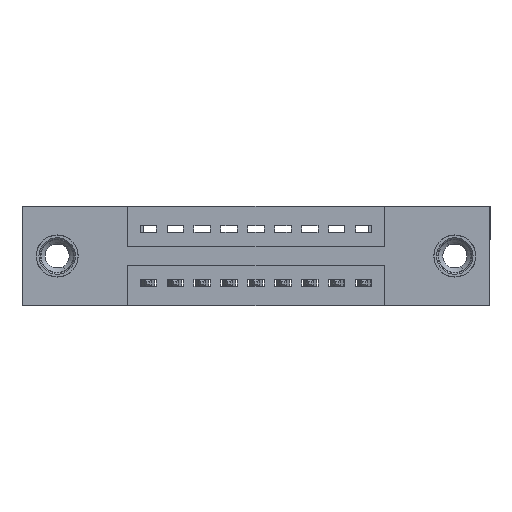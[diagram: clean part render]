
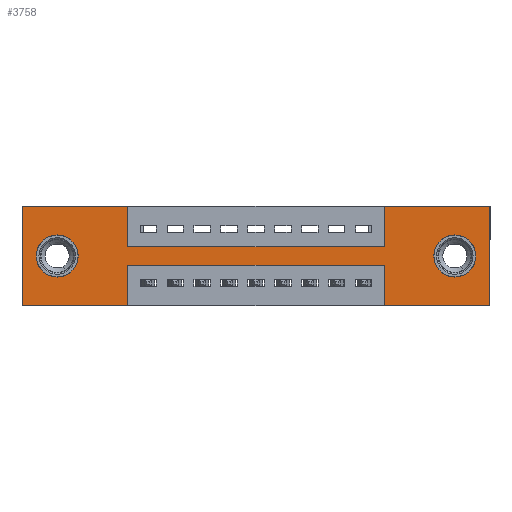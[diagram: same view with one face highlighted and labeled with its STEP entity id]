
A CAD part, front view. The second image highlights one B-rep face of the part: STEP entity #3758.
In plain terms, the highlighted planar face has unit normal (0, -1, 0).
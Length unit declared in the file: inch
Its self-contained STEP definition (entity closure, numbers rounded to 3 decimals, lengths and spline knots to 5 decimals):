
#44 = VECTOR ( 'NONE', #261, 39.37008 ) ;
#188 = VERTEX_POINT ( 'NONE', #5067 ) ;
#201 = EDGE_CURVE ( 'NONE', #7228, #4524, #6579, .T. ) ;
#225 = EDGE_CURVE ( 'NONE', #1121, #188, #7376, .T. ) ;
#253 = ORIENTED_EDGE ( 'NONE', *, *, #12209, .F. ) ;
#261 = DIRECTION ( 'NONE',  ( 0., 0., -1. ) ) ;
#304 = VERTEX_POINT ( 'NONE', #8446 ) ;
#416 = EDGE_CURVE ( 'NONE', #8986, #6465, #934, .T. ) ;
#478 = CARTESIAN_POINT ( 'NONE',  ( 0., 0., 0. ) ) ;
#480 = DIRECTION ( 'NONE',  ( 1., 0., 0. ) ) ;
#505 = LINE ( 'NONE', #9647, #12288 ) ;
#551 = ORIENTED_EDGE ( 'NONE', *, *, #8954, .F. ) ;
#598 = ORIENTED_EDGE ( 'NONE', *, *, #416, .T. ) ;
#721 = CARTESIAN_POINT ( 'NONE',  ( 0.3925, 0., -0.15 ) ) ;
#870 = ORIENTED_EDGE ( 'NONE', *, *, #201, .F. ) ;
#888 = EDGE_CURVE ( 'NONE', #2505, #5016, #10098, .T. ) ;
#934 = CIRCLE ( 'NONE', #12298, 0.078 ) ;
#1121 = VERTEX_POINT ( 'NONE', #9405 ) ;
#1177 = LINE ( 'NONE', #2884, #6327 ) ;
#1178 = EDGE_CURVE ( 'NONE', #2474, #5513, #10087, .T. ) ;
#1232 = CARTESIAN_POINT ( 'NONE',  ( 1.3425, 0., -0.15 ) ) ;
#1363 = LINE ( 'NONE', #12987, #12840 ) ;
#1561 = DIRECTION ( 'NONE',  ( 0., 0., 1. ) ) ;
#1634 = ORIENTED_EDGE ( 'NONE', *, *, #2794, .F. ) ;
#1692 = DIRECTION ( 'NONE',  ( 0., 0., -1. ) ) ;
#1800 = LINE ( 'NONE', #11561, #6954 ) ;
#2004 = DIRECTION ( 'NONE',  ( 0., 0., -1. ) ) ;
#2189 = DIRECTION ( 'NONE',  ( 0., 1., 0. ) ) ;
#2382 = AXIS2_PLACEMENT_3D ( 'NONE', #7420, #2189, #8302 ) ;
#2464 = EDGE_CURVE ( 'NONE', #6863, #6391, #1363, .T. ) ;
#2474 = VERTEX_POINT ( 'NONE', #10670 ) ;
#2505 = VERTEX_POINT ( 'NONE', #6942 ) ;
#2624 = LINE ( 'NONE', #8159, #13284 ) ;
#2680 = ORIENTED_EDGE ( 'NONE', *, *, #2464, .F. ) ;
#2794 = EDGE_CURVE ( 'NONE', #12512, #304, #3774, .T. ) ;
#2876 = CARTESIAN_POINT ( 'NONE',  ( 0.3925, 0., -0.37 ) ) ;
#2884 = CARTESIAN_POINT ( 'NONE',  ( 0., 0., 0. ) ) ;
#2957 = CARTESIAN_POINT ( 'NONE',  ( 0., 0., -0.37 ) ) ;
#3030 = DIRECTION ( 'NONE',  ( 0., 0., -1. ) ) ;
#3136 = VECTOR ( 'NONE', #8350, 39.37008 ) ;
#3281 = ORIENTED_EDGE ( 'NONE', *, *, #9114, .F. ) ;
#3407 = CIRCLE ( 'NONE', #9245, 0.078 ) ;
#3470 = CARTESIAN_POINT ( 'NONE',  ( 0., 0., -0.37 ) ) ;
#3683 = CARTESIAN_POINT ( 'NONE',  ( 1.605, 0., -0.185 ) ) ;
#3758 = ADVANCED_FACE ( 'NONE', ( #7115, #6798, #6649 ), #9208, .T. ) ;
#3774 = LINE ( 'NONE', #12649, #44 ) ;
#3925 = EDGE_CURVE ( 'NONE', #6465, #8986, #5951, .T. ) ;
#3928 = CARTESIAN_POINT ( 'NONE',  ( 1.605, 0., -0.107 ) ) ;
#3933 = ORIENTED_EDGE ( 'NONE', *, *, #9561, .F. ) ;
#4000 = VECTOR ( 'NONE', #10602, 39.37008 ) ;
#4123 = CARTESIAN_POINT ( 'NONE',  ( 0., 0., 0. ) ) ;
#4333 = VECTOR ( 'NONE', #9748, 39.37008 ) ;
#4355 = CARTESIAN_POINT ( 'NONE',  ( 0.3925, 0., 0. ) ) ;
#4524 = VERTEX_POINT ( 'NONE', #8348 ) ;
#4601 = CARTESIAN_POINT ( 'NONE',  ( 0.3925, 0., -0.22 ) ) ;
#4746 = CARTESIAN_POINT ( 'NONE',  ( 1.605, 0., -0.185 ) ) ;
#4803 = CARTESIAN_POINT ( 'NONE',  ( 0.13, 0., -0.185 ) ) ;
#4820 = LINE ( 'NONE', #2876, #8346 ) ;
#5016 = VERTEX_POINT ( 'NONE', #3928 ) ;
#5031 = LINE ( 'NONE', #721, #9381 ) ;
#5067 = CARTESIAN_POINT ( 'NONE',  ( 0., 0., -0.37 ) ) ;
#5081 = DIRECTION ( 'NONE',  ( 0., 0., -1. ) ) ;
#5088 = DIRECTION ( 'NONE',  ( 1., 0., 0. ) ) ;
#5110 = VECTOR ( 'NONE', #1561, 39.37008 ) ;
#5188 = EDGE_LOOP ( 'NONE', ( #9864, #8429 ) ) ;
#5513 = VERTEX_POINT ( 'NONE', #7099 ) ;
#5770 = DIRECTION ( 'NONE',  ( 0., 1., 0. ) ) ;
#5865 = AXIS2_PLACEMENT_3D ( 'NONE', #4746, #6835, #1692 ) ;
#5914 = DIRECTION ( 'NONE',  ( 1., 0., 0. ) ) ;
#5951 = CIRCLE ( 'NONE', #2382, 0.078 ) ;
#6327 = VECTOR ( 'NONE', #5088, 39.37008 ) ;
#6391 = VERTEX_POINT ( 'NONE', #9719 ) ;
#6465 = VERTEX_POINT ( 'NONE', #10808 ) ;
#6498 = EDGE_LOOP ( 'NONE', ( #598, #12131 ) ) ;
#6579 = LINE ( 'NONE', #4601, #4000 ) ;
#6613 = EDGE_CURVE ( 'NONE', #188, #6941, #13375, .T. ) ;
#6649 = FACE_OUTER_BOUND ( 'NONE', #7672, .T. ) ;
#6798 = FACE_BOUND ( 'NONE', #6498, .T. ) ;
#6835 = DIRECTION ( 'NONE',  ( 0., 1., 0. ) ) ;
#6863 = VERTEX_POINT ( 'NONE', #11289 ) ;
#6941 = VERTEX_POINT ( 'NONE', #4123 ) ;
#6942 = CARTESIAN_POINT ( 'NONE',  ( 1.605, 0., -0.263 ) ) ;
#6954 = VECTOR ( 'NONE', #12658, 39.37008 ) ;
#7099 = CARTESIAN_POINT ( 'NONE',  ( 1.3425, 0., -0.37 ) ) ;
#7115 = FACE_BOUND ( 'NONE', #5188, .T. ) ;
#7228 = VERTEX_POINT ( 'NONE', #7607 ) ;
#7376 = LINE ( 'NONE', #3470, #4333 ) ;
#7420 = CARTESIAN_POINT ( 'NONE',  ( 0.13, 0., -0.185 ) ) ;
#7607 = CARTESIAN_POINT ( 'NONE',  ( 1.3425, 0., -0.22 ) ) ;
#7672 = EDGE_LOOP ( 'NONE', ( #253, #870, #7832, #12107, #3933, #2680, #3281, #8566, #1634, #551, #10518, #7903 ) ) ;
#7832 = ORIENTED_EDGE ( 'NONE', *, *, #11456, .F. ) ;
#7903 = ORIENTED_EDGE ( 'NONE', *, *, #225, .F. ) ;
#8159 = CARTESIAN_POINT ( 'NONE',  ( 1.735, 0., 0. ) ) ;
#8302 = DIRECTION ( 'NONE',  ( 0., 0., 1. ) ) ;
#8346 = VECTOR ( 'NONE', #5081, 39.37008 ) ;
#8348 = CARTESIAN_POINT ( 'NONE',  ( 0.3925, 0., -0.22 ) ) ;
#8350 = DIRECTION ( 'NONE',  ( -1., 0., 0. ) ) ;
#8429 = ORIENTED_EDGE ( 'NONE', *, *, #888, .T. ) ;
#8446 = CARTESIAN_POINT ( 'NONE',  ( 0.3925, 0., -0.15 ) ) ;
#8566 = ORIENTED_EDGE ( 'NONE', *, *, #9412, .F. ) ;
#8755 = VERTEX_POINT ( 'NONE', #1232 ) ;
#8786 = DIRECTION ( 'NONE',  ( 0., 0., 1. ) ) ;
#8954 = EDGE_CURVE ( 'NONE', #6941, #12512, #1177, .T. ) ;
#8986 = VERTEX_POINT ( 'NONE', #11293 ) ;
#9114 = EDGE_CURVE ( 'NONE', #8755, #6863, #1800, .T. ) ;
#9208 = PLANE ( 'NONE',  #10697 ) ;
#9245 = AXIS2_PLACEMENT_3D ( 'NONE', #3683, #11915, #9806 ) ;
#9250 = DIRECTION ( 'NONE',  ( 0., -1., 0. ) ) ;
#9381 = VECTOR ( 'NONE', #5914, 39.37008 ) ;
#9405 = CARTESIAN_POINT ( 'NONE',  ( 0.3925, 0., -0.37 ) ) ;
#9412 = EDGE_CURVE ( 'NONE', #304, #8755, #5031, .T. ) ;
#9451 = CARTESIAN_POINT ( 'NONE',  ( 0., 0., -0.37 ) ) ;
#9561 = EDGE_CURVE ( 'NONE', #6391, #2474, #2624, .T. ) ;
#9647 = CARTESIAN_POINT ( 'NONE',  ( 1.3425, 0., -0.37 ) ) ;
#9719 = CARTESIAN_POINT ( 'NONE',  ( 1.735, 0., 0. ) ) ;
#9748 = DIRECTION ( 'NONE',  ( -1., 0., 0. ) ) ;
#9806 = DIRECTION ( 'NONE',  ( 0., 0., -1. ) ) ;
#9864 = ORIENTED_EDGE ( 'NONE', *, *, #9895, .T. ) ;
#9895 = EDGE_CURVE ( 'NONE', #5016, #2505, #3407, .T. ) ;
#10087 = LINE ( 'NONE', #9451, #3136 ) ;
#10098 = CIRCLE ( 'NONE', #5865, 0.078 ) ;
#10518 = ORIENTED_EDGE ( 'NONE', *, *, #6613, .F. ) ;
#10602 = DIRECTION ( 'NONE',  ( -1., 0., 0. ) ) ;
#10670 = CARTESIAN_POINT ( 'NONE',  ( 1.735, 0., -0.37 ) ) ;
#10697 = AXIS2_PLACEMENT_3D ( 'NONE', #2957, #9250, #3030 ) ;
#10808 = CARTESIAN_POINT ( 'NONE',  ( 0.13, 0., -0.263 ) ) ;
#11289 = CARTESIAN_POINT ( 'NONE',  ( 1.3425, 0., 0. ) ) ;
#11293 = CARTESIAN_POINT ( 'NONE',  ( 0.13, 0., -0.107 ) ) ;
#11456 = EDGE_CURVE ( 'NONE', #5513, #7228, #505, .T. ) ;
#11561 = CARTESIAN_POINT ( 'NONE',  ( 1.3425, 0., 0. ) ) ;
#11915 = DIRECTION ( 'NONE',  ( 0., 1., 0. ) ) ;
#12107 = ORIENTED_EDGE ( 'NONE', *, *, #1178, .F. ) ;
#12131 = ORIENTED_EDGE ( 'NONE', *, *, #3925, .T. ) ;
#12209 = EDGE_CURVE ( 'NONE', #4524, #1121, #4820, .T. ) ;
#12288 = VECTOR ( 'NONE', #12847, 39.37008 ) ;
#12298 = AXIS2_PLACEMENT_3D ( 'NONE', #4803, #5770, #8786 ) ;
#12512 = VERTEX_POINT ( 'NONE', #4355 ) ;
#12649 = CARTESIAN_POINT ( 'NONE',  ( 0.3925, 0., 0. ) ) ;
#12658 = DIRECTION ( 'NONE',  ( 0., 0., 1. ) ) ;
#12840 = VECTOR ( 'NONE', #480, 39.37008 ) ;
#12847 = DIRECTION ( 'NONE',  ( 0., 0., 1. ) ) ;
#12987 = CARTESIAN_POINT ( 'NONE',  ( 0., 0., 0. ) ) ;
#13284 = VECTOR ( 'NONE', #2004, 39.37008 ) ;
#13375 = LINE ( 'NONE', #478, #5110 ) ;
